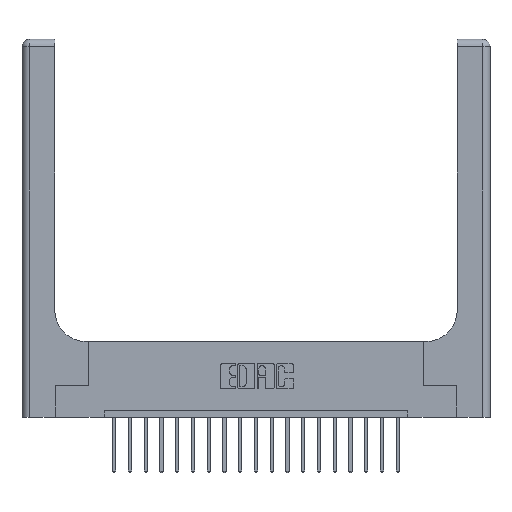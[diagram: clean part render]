
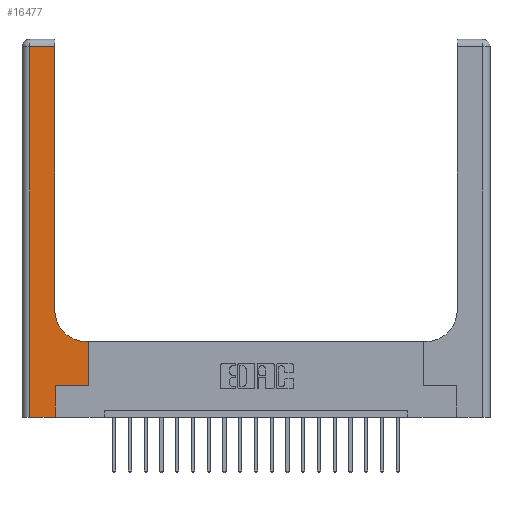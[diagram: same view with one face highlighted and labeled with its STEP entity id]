
A CAD part, top view. The second image highlights one B-rep face of the part: STEP entity #16477.
In plain terms, the highlighted planar face has unit normal (0, 0, 1).
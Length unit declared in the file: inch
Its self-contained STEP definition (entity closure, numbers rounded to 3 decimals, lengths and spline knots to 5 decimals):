
#26 = DIRECTION ( 'NONE',  ( 1., 0., 0. ) ) ;
#364 = LINE ( 'NONE', #4147, #12229 ) ;
#371 = PLANE ( 'NONE',  #3470 ) ;
#646 = EDGE_LOOP ( 'NONE', ( #6783, #15476, #16349, #1096, #8054, #11096, #6817, #1546, #5268 ) ) ;
#833 = LINE ( 'NONE', #18481, #12462 ) ;
#1096 = ORIENTED_EDGE ( 'NONE', *, *, #14971, .T. ) ;
#1500 = CARTESIAN_POINT ( 'NONE',  ( 0., 0., 0.37 ) ) ;
#1546 = ORIENTED_EDGE ( 'NONE', *, *, #13830, .T. ) ;
#1845 = CARTESIAN_POINT ( 'NONE',  ( 0.06, 2.94, 0.37 ) ) ;
#2117 = DIRECTION ( 'NONE',  ( 0., 0., -1. ) ) ;
#3470 = AXIS2_PLACEMENT_3D ( 'NONE', #19088, #6643, #11116 ) ;
#3475 = CIRCLE ( 'NONE', #19879, 0.25 ) ;
#4147 = CARTESIAN_POINT ( 'NONE',  ( 0.265, 0., 0.37 ) ) ;
#4332 = CARTESIAN_POINT ( 'NONE',  ( 0.26, 0.6, 0.37 ) ) ;
#4901 = DIRECTION ( 'NONE',  ( -1., 0., 0. ) ) ;
#5268 = ORIENTED_EDGE ( 'NONE', *, *, #8320, .T. ) ;
#5331 = CARTESIAN_POINT ( 'NONE',  ( 0.51, 0.85, 0.37 ) ) ;
#5842 = LINE ( 'NONE', #17644, #11898 ) ;
#6643 = DIRECTION ( 'NONE',  ( 0., 0., -1. ) ) ;
#6783 = ORIENTED_EDGE ( 'NONE', *, *, #7460, .T. ) ;
#6817 = ORIENTED_EDGE ( 'NONE', *, *, #15023, .T. ) ;
#6978 = LINE ( 'NONE', #15963, #18904 ) ;
#7037 = DIRECTION ( 'NONE',  ( 0., 1., 0. ) ) ;
#7133 = EDGE_CURVE ( 'NONE', #18041, #16318, #364, .T. ) ;
#7460 = EDGE_CURVE ( 'NONE', #19517, #18408, #833, .T. ) ;
#7701 = VERTEX_POINT ( 'NONE', #8338 ) ;
#8054 = ORIENTED_EDGE ( 'NONE', *, *, #7133, .T. ) ;
#8320 = EDGE_CURVE ( 'NONE', #17280, #19517, #3475, .T. ) ;
#8338 = CARTESIAN_POINT ( 'NONE',  ( 0.528, 0.6, 0.37 ) ) ;
#8693 = CARTESIAN_POINT ( 'NONE',  ( 0.51, 0.6, 0.37 ) ) ;
#9187 = VERTEX_POINT ( 'NONE', #17647 ) ;
#10014 = EDGE_CURVE ( 'NONE', #15084, #14241, #5842, .T. ) ;
#10208 = DIRECTION ( 'NONE',  ( 0., -1., 0. ) ) ;
#10607 = LINE ( 'NONE', #4332, #18415 ) ;
#10899 = CARTESIAN_POINT ( 'NONE',  ( 0.265, 0.25, 0.37 ) ) ;
#11096 = ORIENTED_EDGE ( 'NONE', *, *, #13568, .T. ) ;
#11116 = DIRECTION ( 'NONE',  ( -1., 0., 0. ) ) ;
#11898 = VECTOR ( 'NONE', #10208, 39.37008 ) ;
#11970 = DIRECTION ( 'NONE',  ( -1., 0., 0. ) ) ;
#12229 = VECTOR ( 'NONE', #17934, 39.37008 ) ;
#12462 = VECTOR ( 'NONE', #7037, 39.37008 ) ;
#13114 = CARTESIAN_POINT ( 'NONE',  ( 0.06, 0., 0.37 ) ) ;
#13568 = EDGE_CURVE ( 'NONE', #16318, #9187, #6978, .T. ) ;
#13830 = EDGE_CURVE ( 'NONE', #7701, #17280, #10607, .T. ) ;
#14238 = CARTESIAN_POINT ( 'NONE',  ( 0.528, 0.25, 0.37 ) ) ;
#14241 = VERTEX_POINT ( 'NONE', #13114 ) ;
#14467 = CARTESIAN_POINT ( 'NONE',  ( 0., 2.94, 0.37 ) ) ;
#14971 = EDGE_CURVE ( 'NONE', #14241, #18041, #18614, .T. ) ;
#15023 = EDGE_CURVE ( 'NONE', #9187, #7701, #16212, .T. ) ;
#15084 = VERTEX_POINT ( 'NONE', #1845 ) ;
#15476 = ORIENTED_EDGE ( 'NONE', *, *, #19429, .T. ) ;
#15546 = LINE ( 'NONE', #14467, #16529 ) ;
#15714 = VECTOR ( 'NONE', #17192, 39.37008 ) ;
#15963 = CARTESIAN_POINT ( 'NONE',  ( 0.265, 0.25, 0.37 ) ) ;
#16100 = CARTESIAN_POINT ( 'NONE',  ( 0.26, 2.94, 0.37 ) ) ;
#16212 = LINE ( 'NONE', #14238, #15714 ) ;
#16318 = VERTEX_POINT ( 'NONE', #10899 ) ;
#16349 = ORIENTED_EDGE ( 'NONE', *, *, #10014, .T. ) ;
#16477 = ADVANCED_FACE ( 'NONE', ( #17151 ), #371, .F. ) ;
#16529 = VECTOR ( 'NONE', #4901, 39.37008 ) ;
#16730 = CARTESIAN_POINT ( 'NONE',  ( 0.265, 0., 0.37 ) ) ;
#17151 = FACE_OUTER_BOUND ( 'NONE', #646, .T. ) ;
#17192 = DIRECTION ( 'NONE',  ( 0., 1., 0. ) ) ;
#17280 = VERTEX_POINT ( 'NONE', #8693 ) ;
#17432 = CARTESIAN_POINT ( 'NONE',  ( 0.26, 0.85, 0.37 ) ) ;
#17644 = CARTESIAN_POINT ( 'NONE',  ( 0.06, 3., 0.37 ) ) ;
#17647 = CARTESIAN_POINT ( 'NONE',  ( 0.528, 0.25, 0.37 ) ) ;
#17653 = DIRECTION ( 'NONE',  ( 1., 0., 0. ) ) ;
#17711 = DIRECTION ( 'NONE',  ( 1., 0., 0. ) ) ;
#17934 = DIRECTION ( 'NONE',  ( 0., 1., 0. ) ) ;
#18041 = VERTEX_POINT ( 'NONE', #16730 ) ;
#18408 = VERTEX_POINT ( 'NONE', #16100 ) ;
#18415 = VECTOR ( 'NONE', #11970, 39.37008 ) ;
#18481 = CARTESIAN_POINT ( 'NONE',  ( 0.26, 3., 0.37 ) ) ;
#18614 = LINE ( 'NONE', #1500, #19096 ) ;
#18904 = VECTOR ( 'NONE', #17711, 39.37008 ) ;
#19088 = CARTESIAN_POINT ( 'NONE',  ( 0., 3., 0.37 ) ) ;
#19096 = VECTOR ( 'NONE', #26, 39.37008 ) ;
#19429 = EDGE_CURVE ( 'NONE', #18408, #15084, #15546, .T. ) ;
#19517 = VERTEX_POINT ( 'NONE', #17432 ) ;
#19879 = AXIS2_PLACEMENT_3D ( 'NONE', #5331, #2117, #17653 ) ;
